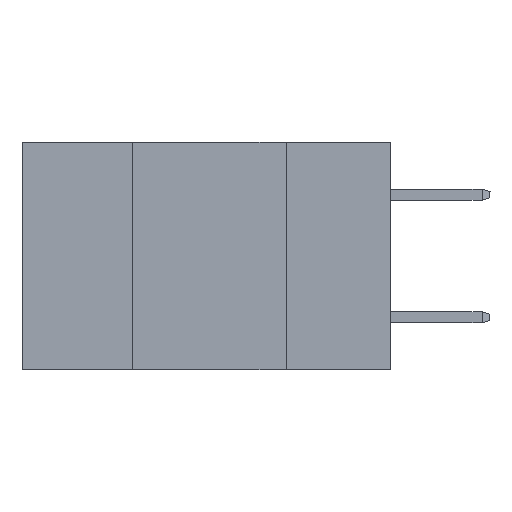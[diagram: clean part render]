
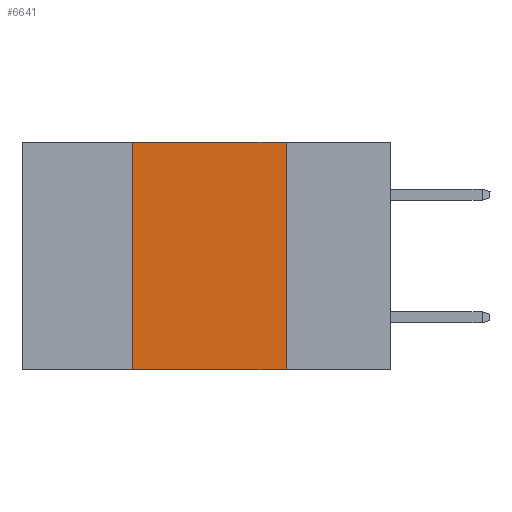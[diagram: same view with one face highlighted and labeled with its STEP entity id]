
A CAD part, left-side view. The second image highlights one B-rep face of the part: STEP entity #6641.
In plain terms, the highlighted planar face has unit normal (-1, 0, 0).
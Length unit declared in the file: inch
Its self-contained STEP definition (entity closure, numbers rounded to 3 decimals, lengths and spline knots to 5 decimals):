
#696 = VERTEX_POINT ( 'NONE', #10055 ) ;
#832 = LINE ( 'NONE', #8840, #5202 ) ;
#836 = EDGE_LOOP ( 'NONE', ( #21186, #21589, #18453, #9840 ) ) ;
#958 = LINE ( 'NONE', #984, #21965 ) ;
#984 = CARTESIAN_POINT ( 'NONE',  ( 0., 0.6, 0. ) ) ;
#1064 = DIRECTION ( 'NONE',  ( 0., -1., 0. ) ) ;
#3966 = DIRECTION ( 'NONE',  ( 0., 0., -1. ) ) ;
#4081 = VERTEX_POINT ( 'NONE', #9927 ) ;
#5022 = LINE ( 'NONE', #13587, #17899 ) ;
#5202 = VECTOR ( 'NONE', #18633, 39.37008 ) ;
#5833 = VECTOR ( 'NONE', #3966, 39.37008 ) ;
#6124 = EDGE_CURVE ( 'NONE', #4081, #11959, #958, .T. ) ;
#6167 = CARTESIAN_POINT ( 'NONE',  ( 0., 0.17, 0. ) ) ;
#6601 = CARTESIAN_POINT ( 'NONE',  ( 0., 0.6, 0. ) ) ;
#6641 = ADVANCED_FACE ( 'NONE', ( #17646 ), #11690, .F. ) ;
#6996 = EDGE_CURVE ( 'NONE', #11959, #13394, #10502, .T. ) ;
#8372 = DIRECTION ( 'NONE',  ( 1., 0., 0. ) ) ;
#8742 = EDGE_CURVE ( 'NONE', #696, #4081, #832, .T. ) ;
#8840 = CARTESIAN_POINT ( 'NONE',  ( 0., 0.42, 0. ) ) ;
#9174 = CARTESIAN_POINT ( 'NONE',  ( 0., 0.17, -0.37 ) ) ;
#9840 = ORIENTED_EDGE ( 'NONE', *, *, #12664, .T. ) ;
#9927 = CARTESIAN_POINT ( 'NONE',  ( 0., 0.42, 0. ) ) ;
#10055 = CARTESIAN_POINT ( 'NONE',  ( 0., 0.42, -0.37 ) ) ;
#10502 = LINE ( 'NONE', #17433, #5833 ) ;
#11690 = PLANE ( 'NONE',  #16567 ) ;
#11959 = VERTEX_POINT ( 'NONE', #6167 ) ;
#12664 = EDGE_CURVE ( 'NONE', #696, #13394, #5022, .T. ) ;
#13394 = VERTEX_POINT ( 'NONE', #9174 ) ;
#13587 = CARTESIAN_POINT ( 'NONE',  ( 0., 0.6, -0.37 ) ) ;
#16567 = AXIS2_PLACEMENT_3D ( 'NONE', #6601, #8372, #19836 ) ;
#16862 = DIRECTION ( 'NONE',  ( 0., -1., 0. ) ) ;
#17433 = CARTESIAN_POINT ( 'NONE',  ( 0., 0.17, 0. ) ) ;
#17646 = FACE_OUTER_BOUND ( 'NONE', #836, .T. ) ;
#17899 = VECTOR ( 'NONE', #16862, 39.37008 ) ;
#18453 = ORIENTED_EDGE ( 'NONE', *, *, #8742, .F. ) ;
#18633 = DIRECTION ( 'NONE',  ( 0., 0., 1. ) ) ;
#19836 = DIRECTION ( 'NONE',  ( 0., 0., -1. ) ) ;
#21186 = ORIENTED_EDGE ( 'NONE', *, *, #6996, .F. ) ;
#21589 = ORIENTED_EDGE ( 'NONE', *, *, #6124, .F. ) ;
#21965 = VECTOR ( 'NONE', #1064, 39.37008 ) ;
